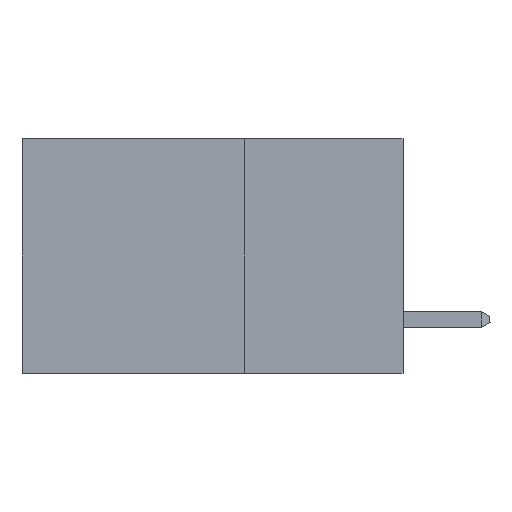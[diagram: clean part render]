
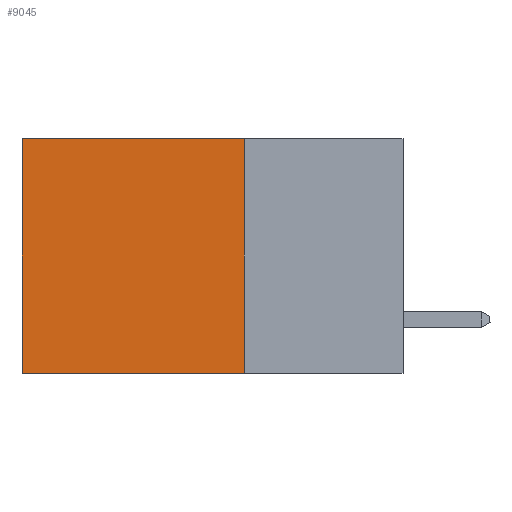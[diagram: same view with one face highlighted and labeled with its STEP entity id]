
A CAD part, left-side view. The second image highlights one B-rep face of the part: STEP entity #9045.
In plain terms, the highlighted planar face has unit normal (-1, 0, 0).
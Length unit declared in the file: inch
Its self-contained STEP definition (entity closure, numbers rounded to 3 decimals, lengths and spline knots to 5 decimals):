
#1119 = LINE ( 'NONE', #12454, #1940 ) ;
#1180 = LINE ( 'NONE', #10628, #4998 ) ;
#1185 = VERTEX_POINT ( 'NONE', #7497 ) ;
#1661 = EDGE_CURVE ( 'NONE', #9595, #8740, #5260, .T. ) ;
#1940 = VECTOR ( 'NONE', #6318, 39.37008 ) ;
#1944 = ORIENTED_EDGE ( 'NONE', *, *, #13232, .F. ) ;
#3134 = AXIS2_PLACEMENT_3D ( 'NONE', #5215, #12770, #4283 ) ;
#3222 = PLANE ( 'NONE',  #3134 ) ;
#4283 = DIRECTION ( 'NONE',  ( 0., 0., -1. ) ) ;
#4679 = LINE ( 'NONE', #10092, #5547 ) ;
#4998 = VECTOR ( 'NONE', #10537, 39.37008 ) ;
#5215 = CARTESIAN_POINT ( 'NONE',  ( 0.2875, 0.25, 0. ) ) ;
#5249 = ORIENTED_EDGE ( 'NONE', *, *, #8361, .T. ) ;
#5260 = LINE ( 'NONE', #13603, #6725 ) ;
#5372 = DIRECTION ( 'NONE',  ( 0., 1., 0. ) ) ;
#5547 = VECTOR ( 'NONE', #9129, 39.37008 ) ;
#6224 = VERTEX_POINT ( 'NONE', #12866 ) ;
#6318 = DIRECTION ( 'NONE',  ( 0., 0., -1. ) ) ;
#6725 = VECTOR ( 'NONE', #5372, 39.37008 ) ;
#7451 = FACE_OUTER_BOUND ( 'NONE', #12791, .T. ) ;
#7497 = CARTESIAN_POINT ( 'NONE',  ( 0.2875, 0.6, 0. ) ) ;
#8105 = ORIENTED_EDGE ( 'NONE', *, *, #1661, .F. ) ;
#8112 = CARTESIAN_POINT ( 'NONE',  ( 0.2875, 0.25, -0.37 ) ) ;
#8272 = ORIENTED_EDGE ( 'NONE', *, *, #10686, .T. ) ;
#8361 = EDGE_CURVE ( 'NONE', #6224, #1185, #1180, .T. ) ;
#8681 = CARTESIAN_POINT ( 'NONE',  ( 0.2875, 0.6, -0.37 ) ) ;
#8740 = VERTEX_POINT ( 'NONE', #8681 ) ;
#9045 = ADVANCED_FACE ( 'NONE', ( #7451 ), #3222, .F. ) ;
#9129 = DIRECTION ( 'NONE',  ( 0., 0., -1. ) ) ;
#9595 = VERTEX_POINT ( 'NONE', #8112 ) ;
#10092 = CARTESIAN_POINT ( 'NONE',  ( 0.2875, 0.25, 0. ) ) ;
#10537 = DIRECTION ( 'NONE',  ( 0., 1., 0. ) ) ;
#10628 = CARTESIAN_POINT ( 'NONE',  ( 0.2875, 0.25, 0. ) ) ;
#10686 = EDGE_CURVE ( 'NONE', #1185, #8740, #1119, .T. ) ;
#12454 = CARTESIAN_POINT ( 'NONE',  ( 0.2875, 0.6, 0. ) ) ;
#12770 = DIRECTION ( 'NONE',  ( 1., 0., 0. ) ) ;
#12791 = EDGE_LOOP ( 'NONE', ( #8272, #8105, #1944, #5249 ) ) ;
#12866 = CARTESIAN_POINT ( 'NONE',  ( 0.2875, 0.25, 0. ) ) ;
#13232 = EDGE_CURVE ( 'NONE', #6224, #9595, #4679, .T. ) ;
#13603 = CARTESIAN_POINT ( 'NONE',  ( 0.2875, 0.25, -0.37 ) ) ;
